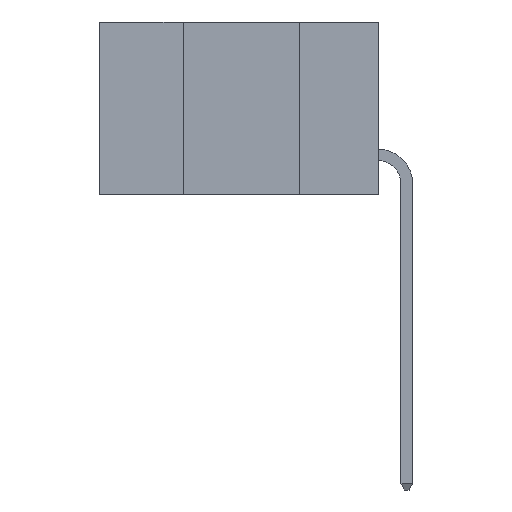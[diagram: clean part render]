
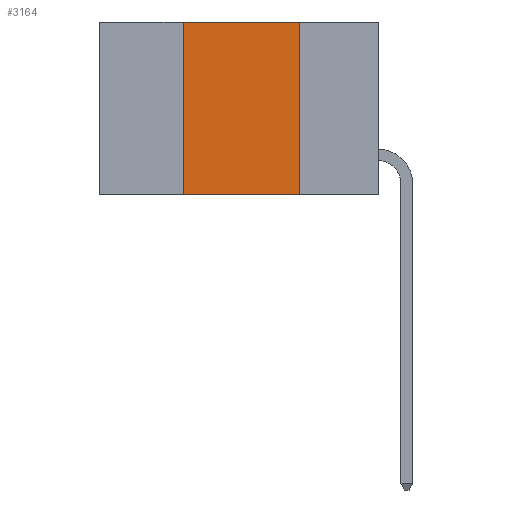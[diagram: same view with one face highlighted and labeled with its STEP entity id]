
A CAD part, left-side view. The second image highlights one B-rep face of the part: STEP entity #3164.
In plain terms, the highlighted planar face has unit normal (-1, 0, 0).
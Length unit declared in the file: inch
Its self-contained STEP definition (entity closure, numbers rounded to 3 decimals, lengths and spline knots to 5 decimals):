
#182 = DIRECTION ( 'NONE',  ( 0., 0., -1. ) ) ;
#345 = CARTESIAN_POINT ( 'NONE',  ( 0., 0.17, -0.37 ) ) ;
#481 = CARTESIAN_POINT ( 'NONE',  ( 0., 0.6, 0. ) ) ;
#1011 = CARTESIAN_POINT ( 'NONE',  ( 0., 0.42, -0.37 ) ) ;
#1093 = CARTESIAN_POINT ( 'NONE',  ( 0., 0.17, 0. ) ) ;
#1135 = CARTESIAN_POINT ( 'NONE',  ( 0., 0.6, -0.37 ) ) ;
#1190 = DIRECTION ( 'NONE',  ( 0., -1., 0. ) ) ;
#1386 = DIRECTION ( 'NONE',  ( 0., 0., -1. ) ) ;
#1543 = DIRECTION ( 'NONE',  ( 0., -1., 0. ) ) ;
#1798 = EDGE_CURVE ( 'NONE', #9894, #11539, #1805, .T. ) ;
#1805 = LINE ( 'NONE', #1135, #10545 ) ;
#2096 = EDGE_CURVE ( 'NONE', #4388, #11539, #3754, .T. ) ;
#2245 = CARTESIAN_POINT ( 'NONE',  ( 0., 0.6, 0. ) ) ;
#2730 = DIRECTION ( 'NONE',  ( 0., 0., 1. ) ) ;
#2749 = ORIENTED_EDGE ( 'NONE', *, *, #12568, .F. ) ;
#3164 = ADVANCED_FACE ( 'NONE', ( #6021 ), #12751, .F. ) ;
#3204 = LINE ( 'NONE', #481, #10990 ) ;
#3403 = ORIENTED_EDGE ( 'NONE', *, *, #9639, .F. ) ;
#3732 = ORIENTED_EDGE ( 'NONE', *, *, #1798, .T. ) ;
#3754 = LINE ( 'NONE', #345, #9058 ) ;
#3777 = CARTESIAN_POINT ( 'NONE',  ( 0., 0.42, -0.37 ) ) ;
#4388 = VERTEX_POINT ( 'NONE', #1093 ) ;
#4416 = VERTEX_POINT ( 'NONE', #10659 ) ;
#5156 = AXIS2_PLACEMENT_3D ( 'NONE', #2245, #6445, #182 ) ;
#5198 = ORIENTED_EDGE ( 'NONE', *, *, #2096, .F. ) ;
#6021 = FACE_OUTER_BOUND ( 'NONE', #7326, .T. ) ;
#6445 = DIRECTION ( 'NONE',  ( 1., 0., 0. ) ) ;
#6894 = LINE ( 'NONE', #3777, #12172 ) ;
#7326 = EDGE_LOOP ( 'NONE', ( #5198, #2749, #3403, #3732 ) ) ;
#9058 = VECTOR ( 'NONE', #1386, 39.37008 ) ;
#9639 = EDGE_CURVE ( 'NONE', #9894, #4416, #6894, .T. ) ;
#9894 = VERTEX_POINT ( 'NONE', #1011 ) ;
#10545 = VECTOR ( 'NONE', #1190, 39.37008 ) ;
#10659 = CARTESIAN_POINT ( 'NONE',  ( 0., 0.42, 0. ) ) ;
#10990 = VECTOR ( 'NONE', #1543, 39.37008 ) ;
#11216 = CARTESIAN_POINT ( 'NONE',  ( 0., 0.17, -0.37 ) ) ;
#11539 = VERTEX_POINT ( 'NONE', #11216 ) ;
#12172 = VECTOR ( 'NONE', #2730, 39.37008 ) ;
#12568 = EDGE_CURVE ( 'NONE', #4416, #4388, #3204, .T. ) ;
#12751 = PLANE ( 'NONE',  #5156 ) ;
